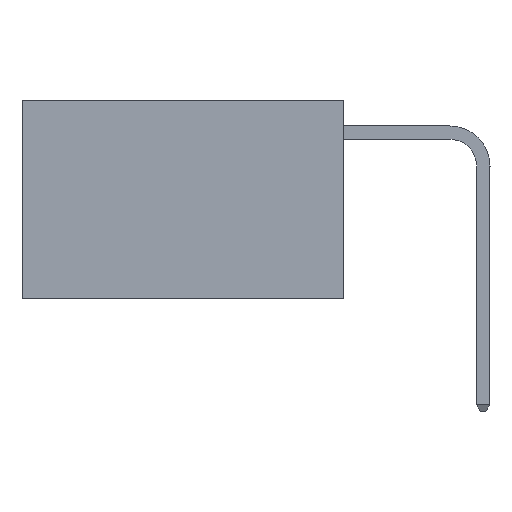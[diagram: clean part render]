
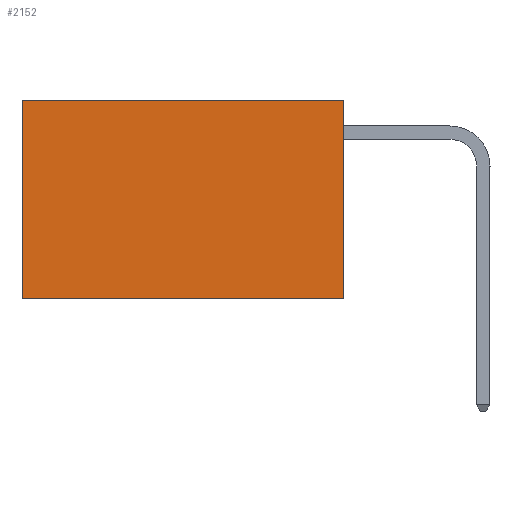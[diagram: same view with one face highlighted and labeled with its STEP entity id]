
A CAD part, left-side view. The second image highlights one B-rep face of the part: STEP entity #2152.
In plain terms, the highlighted planar face has unit normal (-1, 0, 0).
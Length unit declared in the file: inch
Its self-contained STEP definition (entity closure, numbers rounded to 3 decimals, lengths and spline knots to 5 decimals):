
#1221 = EDGE_CURVE ( 'NONE', #3988, #17526, #24078, .T. ) ;
#1715 = CARTESIAN_POINT ( 'NONE',  ( 0.2625, 0.6, -0.37 ) ) ;
#2152 = ADVANCED_FACE ( 'NONE', ( #6219 ), #13940, .F. ) ;
#3988 = VERTEX_POINT ( 'NONE', #9650 ) ;
#5699 = DIRECTION ( 'NONE',  ( 0., 0., -1. ) ) ;
#6219 = FACE_OUTER_BOUND ( 'NONE', #13789, .T. ) ;
#7960 = CARTESIAN_POINT ( 'NONE',  ( 0.2625, 0., 0. ) ) ;
#8610 = EDGE_CURVE ( 'NONE', #10341, #3988, #24076, .T. ) ;
#9650 = CARTESIAN_POINT ( 'NONE',  ( 0.2625, 0., -0.37 ) ) ;
#10341 = VERTEX_POINT ( 'NONE', #22108 ) ;
#10655 = DIRECTION ( 'NONE',  ( 0., 1., 0. ) ) ;
#11576 = CARTESIAN_POINT ( 'NONE',  ( 0.2625, 0.6, 0. ) ) ;
#13571 = EDGE_CURVE ( 'NONE', #15936, #17526, #19908, .T. ) ;
#13789 = EDGE_LOOP ( 'NONE', ( #25382, #20370, #20325, #15995 ) ) ;
#13940 = PLANE ( 'NONE',  #21930 ) ;
#14304 = DIRECTION ( 'NONE',  ( 0., 1., 0. ) ) ;
#15936 = VERTEX_POINT ( 'NONE', #11576 ) ;
#15995 = ORIENTED_EDGE ( 'NONE', *, *, #22242, .T. ) ;
#15996 = CARTESIAN_POINT ( 'NONE',  ( 0.2625, 0., 0. ) ) ;
#16034 = LINE ( 'NONE', #23009, #21595 ) ;
#16062 = DIRECTION ( 'NONE',  ( 0., 0., -1. ) ) ;
#17526 = VERTEX_POINT ( 'NONE', #1715 ) ;
#18076 = DIRECTION ( 'NONE',  ( 1., 0., 0. ) ) ;
#18560 = VECTOR ( 'NONE', #14304, 39.37008 ) ;
#19908 = LINE ( 'NONE', #22357, #24720 ) ;
#20325 = ORIENTED_EDGE ( 'NONE', *, *, #8610, .F. ) ;
#20370 = ORIENTED_EDGE ( 'NONE', *, *, #1221, .F. ) ;
#21595 = VECTOR ( 'NONE', #10655, 39.37008 ) ;
#21930 = AXIS2_PLACEMENT_3D ( 'NONE', #15996, #18076, #5699 ) ;
#22108 = CARTESIAN_POINT ( 'NONE',  ( 0.2625, 0., 0. ) ) ;
#22242 = EDGE_CURVE ( 'NONE', #10341, #15936, #16034, .T. ) ;
#22357 = CARTESIAN_POINT ( 'NONE',  ( 0.2625, 0.6, 0. ) ) ;
#23009 = CARTESIAN_POINT ( 'NONE',  ( 0.2625, 0., 0. ) ) ;
#23382 = CARTESIAN_POINT ( 'NONE',  ( 0.2625, 0., -0.37 ) ) ;
#23447 = VECTOR ( 'NONE', #24570, 39.37008 ) ;
#24076 = LINE ( 'NONE', #7960, #23447 ) ;
#24078 = LINE ( 'NONE', #23382, #18560 ) ;
#24570 = DIRECTION ( 'NONE',  ( 0., 0., -1. ) ) ;
#24720 = VECTOR ( 'NONE', #16062, 39.37008 ) ;
#25382 = ORIENTED_EDGE ( 'NONE', *, *, #13571, .T. ) ;
